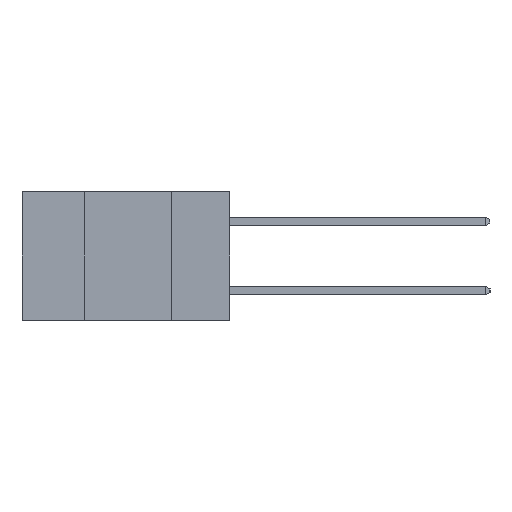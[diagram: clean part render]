
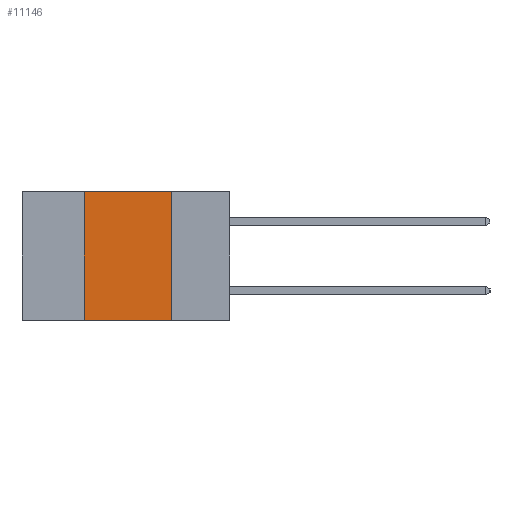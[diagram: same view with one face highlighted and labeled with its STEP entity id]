
A CAD part, left-side view. The second image highlights one B-rep face of the part: STEP entity #11146.
In plain terms, the highlighted planar face has unit normal (-1, 0, 0).
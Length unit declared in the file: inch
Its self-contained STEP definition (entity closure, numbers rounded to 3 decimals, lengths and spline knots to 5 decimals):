
#2 = VECTOR ( 'NONE', #2671, 39.37008 ) ;
#504 = ORIENTED_EDGE ( 'NONE', *, *, #7074, .F. ) ;
#796 = VECTOR ( 'NONE', #3823, 39.37008 ) ;
#1318 = EDGE_CURVE ( 'NONE', #1550, #5414, #1776, .T. ) ;
#1331 = VECTOR ( 'NONE', #8512, 39.37008 ) ;
#1550 = VERTEX_POINT ( 'NONE', #16146 ) ;
#1696 = PLANE ( 'NONE',  #9859 ) ;
#1776 = LINE ( 'NONE', #15530, #1331 ) ;
#1849 = EDGE_LOOP ( 'NONE', ( #7018, #504, #17645, #4603 ) ) ;
#2156 = CARTESIAN_POINT ( 'NONE',  ( 0., 0.17, -0.37 ) ) ;
#2288 = EDGE_CURVE ( 'NONE', #1550, #10850, #16490, .T. ) ;
#2356 = CARTESIAN_POINT ( 'NONE',  ( 0., 0.17, -0.37 ) ) ;
#2671 = DIRECTION ( 'NONE',  ( 0., -1., 0. ) ) ;
#3166 = DIRECTION ( 'NONE',  ( 0., 0., -1. ) ) ;
#3823 = DIRECTION ( 'NONE',  ( 0., 0., -1. ) ) ;
#4603 = ORIENTED_EDGE ( 'NONE', *, *, #1318, .T. ) ;
#5414 = VERTEX_POINT ( 'NONE', #2156 ) ;
#5544 = VECTOR ( 'NONE', #14185, 39.37008 ) ;
#6408 = LINE ( 'NONE', #2356, #796 ) ;
#7018 = ORIENTED_EDGE ( 'NONE', *, *, #12599, .F. ) ;
#7074 = EDGE_CURVE ( 'NONE', #10850, #10040, #11716, .T. ) ;
#7372 = CARTESIAN_POINT ( 'NONE',  ( 0., 0.42, -0.37 ) ) ;
#8186 = CARTESIAN_POINT ( 'NONE',  ( 0., 0.42, 0. ) ) ;
#8512 = DIRECTION ( 'NONE',  ( 0., -1., 0. ) ) ;
#9859 = AXIS2_PLACEMENT_3D ( 'NONE', #10173, #11544, #3166 ) ;
#10040 = VERTEX_POINT ( 'NONE', #11984 ) ;
#10173 = CARTESIAN_POINT ( 'NONE',  ( 0., 0.6, 0. ) ) ;
#10850 = VERTEX_POINT ( 'NONE', #8186 ) ;
#11146 = ADVANCED_FACE ( 'NONE', ( #17549 ), #1696, .F. ) ;
#11544 = DIRECTION ( 'NONE',  ( 1., 0., 0. ) ) ;
#11716 = LINE ( 'NONE', #17771, #2 ) ;
#11984 = CARTESIAN_POINT ( 'NONE',  ( 0., 0.17, 0. ) ) ;
#12599 = EDGE_CURVE ( 'NONE', #10040, #5414, #6408, .T. ) ;
#14185 = DIRECTION ( 'NONE',  ( 0., 0., 1. ) ) ;
#15530 = CARTESIAN_POINT ( 'NONE',  ( 0., 0.6, -0.37 ) ) ;
#16146 = CARTESIAN_POINT ( 'NONE',  ( 0., 0.42, -0.37 ) ) ;
#16490 = LINE ( 'NONE', #7372, #5544 ) ;
#17549 = FACE_OUTER_BOUND ( 'NONE', #1849, .T. ) ;
#17645 = ORIENTED_EDGE ( 'NONE', *, *, #2288, .F. ) ;
#17771 = CARTESIAN_POINT ( 'NONE',  ( 0., 0.6, 0. ) ) ;
